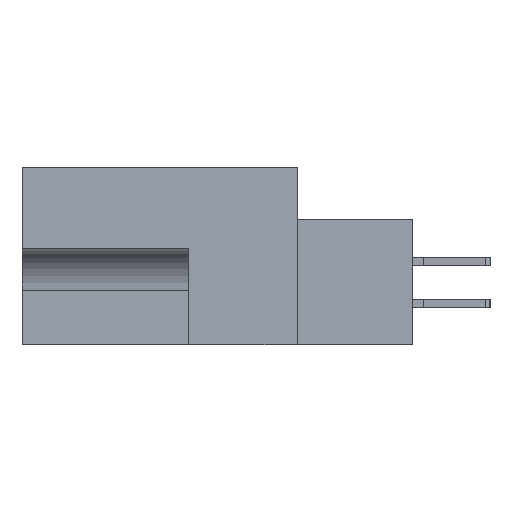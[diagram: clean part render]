
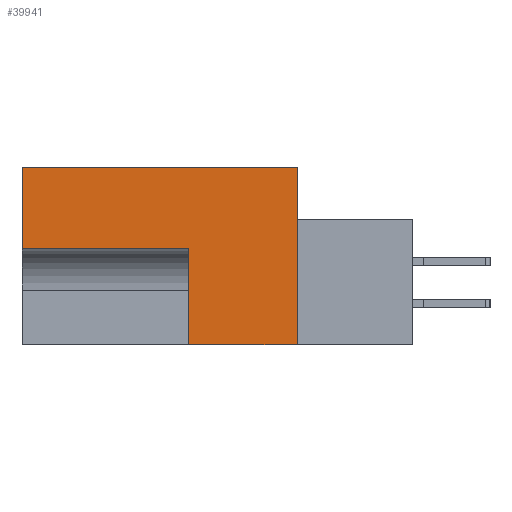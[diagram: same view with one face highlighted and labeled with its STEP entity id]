
A CAD part, left-side view. The second image highlights one B-rep face of the part: STEP entity #39941.
In plain terms, the highlighted planar face has unit normal (-1, 0, 0).
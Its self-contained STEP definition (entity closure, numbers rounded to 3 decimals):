
#194 = VECTOR ( 'NONE', #23693, 1000. ) ;
#602 = LINE ( 'NONE', #14778, #25679 ) ;
#1156 = PLANE ( 'NONE',  #2270 ) ;
#1309 = LINE ( 'NONE', #2341, #194 ) ;
#1841 = ORIENTED_EDGE ( 'NONE', *, *, #45164, .F. ) ;
#2270 = AXIS2_PLACEMENT_3D ( 'NONE', #29838, #33583, #16145 ) ;
#2341 = CARTESIAN_POINT ( 'NONE',  ( 0., 8.255, -13.487 ) ) ;
#2783 = ORIENTED_EDGE ( 'NONE', *, *, #27704, .F. ) ;
#4025 = ORIENTED_EDGE ( 'NONE', *, *, #14187, .F. ) ;
#7492 = EDGE_CURVE ( 'NONE', #19276, #18523, #29236, .T. ) ;
#8561 = VECTOR ( 'NONE', #36746, 1000. ) ;
#9569 = CARTESIAN_POINT ( 'NONE',  ( 0., 8.255, -6.172 ) ) ;
#9738 = VERTEX_POINT ( 'NONE', #45843 ) ;
#10002 = VERTEX_POINT ( 'NONE', #9569 ) ;
#10333 = EDGE_LOOP ( 'NONE', ( #34034, #1841, #4025, #42355, #17476, #2783 ) ) ;
#14058 = FACE_OUTER_BOUND ( 'NONE', #10333, .T. ) ;
#14187 = EDGE_CURVE ( 'NONE', #18177, #9738, #20614, .T. ) ;
#14778 = CARTESIAN_POINT ( 'NONE',  ( 0., 0., 0. ) ) ;
#16044 = DIRECTION ( 'NONE',  ( 0., 1., 0. ) ) ;
#16145 = DIRECTION ( 'NONE',  ( 0., 0., -1. ) ) ;
#17476 = ORIENTED_EDGE ( 'NONE', *, *, #18016, .F. ) ;
#18016 = EDGE_CURVE ( 'NONE', #10002, #26633, #37679, .T. ) ;
#18177 = VERTEX_POINT ( 'NONE', #28807 ) ;
#18523 = VERTEX_POINT ( 'NONE', #45337 ) ;
#18555 = CARTESIAN_POINT ( 'NONE',  ( 0., 20.955, -13.487 ) ) ;
#18954 = CARTESIAN_POINT ( 'NONE',  ( 0., 20.955, -6.172 ) ) ;
#19276 = VERTEX_POINT ( 'NONE', #24877 ) ;
#20614 = LINE ( 'NONE', #39191, #26212 ) ;
#23174 = CARTESIAN_POINT ( 'NONE',  ( 0., 8.255, -6.172 ) ) ;
#23693 = DIRECTION ( 'NONE',  ( 0., 0., 1. ) ) ;
#24877 = CARTESIAN_POINT ( 'NONE',  ( 0., 0., -13.487 ) ) ;
#25679 = VECTOR ( 'NONE', #32683, 1000. ) ;
#26212 = VECTOR ( 'NONE', #42801, 1000. ) ;
#26633 = VERTEX_POINT ( 'NONE', #18954 ) ;
#27704 = EDGE_CURVE ( 'NONE', #18523, #10002, #1309, .T. ) ;
#28807 = CARTESIAN_POINT ( 'NONE',  ( 0., 20.955, 0. ) ) ;
#29236 = LINE ( 'NONE', #45025, #8561 ) ;
#29838 = CARTESIAN_POINT ( 'NONE',  ( 0., 0., 0. ) ) ;
#32683 = DIRECTION ( 'NONE',  ( 0., 0., -1. ) ) ;
#32826 = EDGE_CURVE ( 'NONE', #26633, #18177, #35884, .T. ) ;
#33583 = DIRECTION ( 'NONE',  ( 1., 0., 0. ) ) ;
#34034 = ORIENTED_EDGE ( 'NONE', *, *, #7492, .F. ) ;
#34220 = VECTOR ( 'NONE', #43533, 1000. ) ;
#34849 = VECTOR ( 'NONE', #16044, 1000. ) ;
#35884 = LINE ( 'NONE', #18555, #34220 ) ;
#36746 = DIRECTION ( 'NONE',  ( 0., 1., 0. ) ) ;
#37679 = LINE ( 'NONE', #23174, #34849 ) ;
#39191 = CARTESIAN_POINT ( 'NONE',  ( 0., 11.506, 0. ) ) ;
#39941 = ADVANCED_FACE ( 'NONE', ( #14058 ), #1156, .F. ) ;
#42355 = ORIENTED_EDGE ( 'NONE', *, *, #32826, .F. ) ;
#42801 = DIRECTION ( 'NONE',  ( 0., -1., 0. ) ) ;
#43533 = DIRECTION ( 'NONE',  ( 0., 0., 1. ) ) ;
#45025 = CARTESIAN_POINT ( 'NONE',  ( 0., -8.814, -13.487 ) ) ;
#45164 = EDGE_CURVE ( 'NONE', #9738, #19276, #602, .T. ) ;
#45337 = CARTESIAN_POINT ( 'NONE',  ( 0., 8.255, -13.487 ) ) ;
#45843 = CARTESIAN_POINT ( 'NONE',  ( 0., 0., 0. ) ) ;
